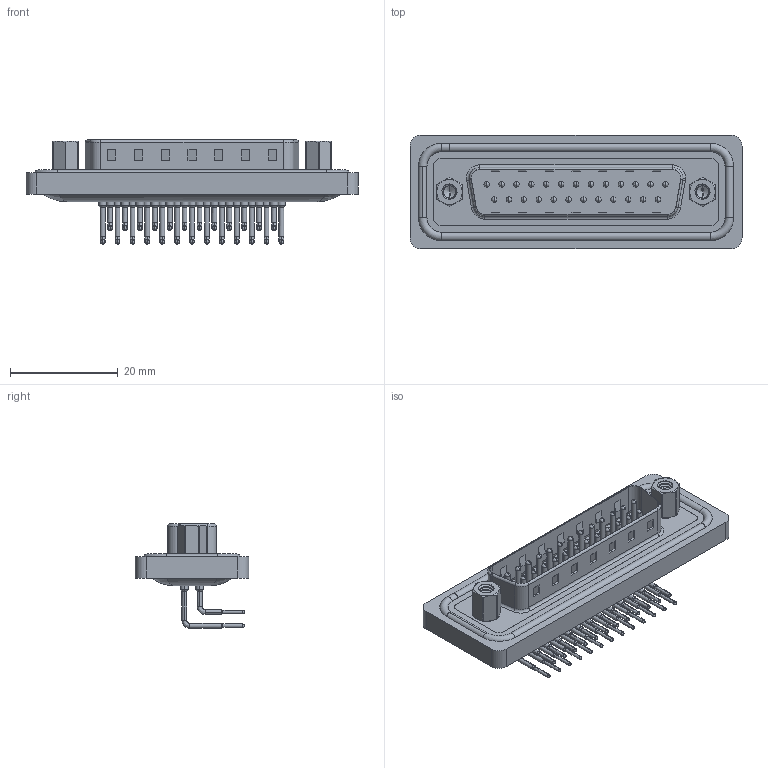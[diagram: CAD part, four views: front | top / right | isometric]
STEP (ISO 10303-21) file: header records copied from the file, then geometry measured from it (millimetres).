
FILE_DESCRIPTION (( 'STEP AP203' ), '1' );
FILE_NAME ('629-W25-340-012.STEP', '2018-11-27T15:46:43', ( '' ), ( '' ), 'SwSTEP 2.0', 'SolidWorks 2016', '' );
FILE_SCHEMA (( 'CONFIG_CONTROL_DESIGN' ));
Length unit declared in the file: millimetre
Products named in the file (8): 629W Shell_25 Contacts; 629W Waterproof Housing_25 Contacts; 629W Contact Row 1; 629W Contact Row 2; 629W 4-40 Threaded Rivet_Stabilizer; 629W 4-40 Hex Standoff; 629-W25-340-012; 629W Housing_25 Contacts
Assembly tree (32 placements, depth 2):
  629-W25-340-012
    629W Housing_25 Contacts
    629W Shell_25 Contacts
    629W Waterproof Housing_25 Contacts
    629W Contact Row 1  x13
    629W Contact Row 2  x12
    629W 4-40 Threaded Rivet_Stabilizer  x2
    629W 4-40 Hex Standoff  x2
Bounding box: 61.74 x 21.1 x 19.39 mm (x, y, z)
Volume: 6441 mm3; surface area: 11482 mm2
Topology: 33 solids, 33 shells, 3312 faces, 9256 edges, 6021 vertices
Faces by surface type: plane 1805, cylinder 1162, bspline 172, cone 130, torus 43
Entity records: 32982 total; most frequent: CARTESIAN_POINT 9388, DIRECTION 4749, ORIENTED_EDGE 4510, EDGE_CURVE 2255, AXIS2_PLACEMENT_3D 1750, VERTEX_POINT 1467, VECTOR 1249, LINE 1249
